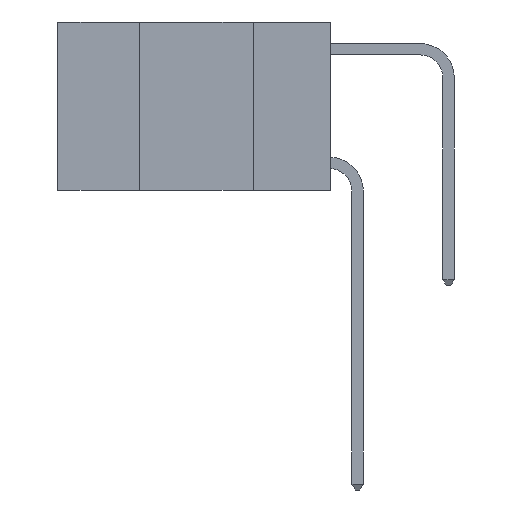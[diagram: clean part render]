
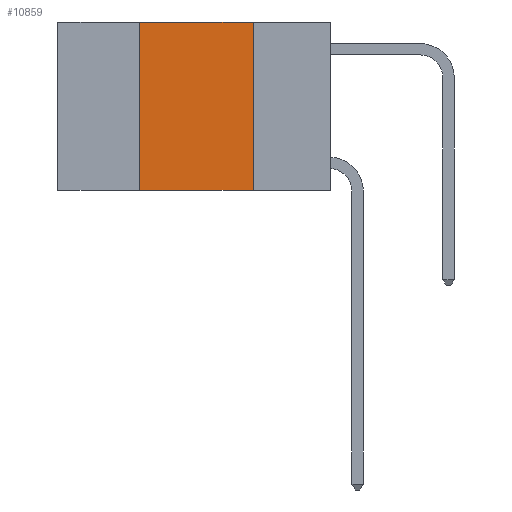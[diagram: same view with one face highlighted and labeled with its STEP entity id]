
A CAD part, left-side view. The second image highlights one B-rep face of the part: STEP entity #10859.
In plain terms, the highlighted planar face has unit normal (-1, 0, 0).
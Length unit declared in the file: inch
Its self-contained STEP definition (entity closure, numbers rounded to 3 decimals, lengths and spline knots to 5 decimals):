
#292 = DIRECTION ( 'NONE',  ( 0., -1., 0. ) ) ;
#1129 = CARTESIAN_POINT ( 'NONE',  ( 0., 0.6, 0. ) ) ;
#1498 = DIRECTION ( 'NONE',  ( 0., -1., 0. ) ) ;
#1882 = VERTEX_POINT ( 'NONE', #3026 ) ;
#1991 = CARTESIAN_POINT ( 'NONE',  ( 0., 0.17, 0. ) ) ;
#2131 = VECTOR ( 'NONE', #7748, 39.37008 ) ;
#3026 = CARTESIAN_POINT ( 'NONE',  ( 0., 0.17, -0.37 ) ) ;
#3060 = VERTEX_POINT ( 'NONE', #3488 ) ;
#3488 = CARTESIAN_POINT ( 'NONE',  ( 0., 0.42, 0. ) ) ;
#3491 = EDGE_CURVE ( 'NONE', #3060, #4662, #6987, .T. ) ;
#3756 = VECTOR ( 'NONE', #1498, 39.37008 ) ;
#3855 = FACE_OUTER_BOUND ( 'NONE', #8008, .T. ) ;
#4045 = LINE ( 'NONE', #7292, #3756 ) ;
#4110 = DIRECTION ( 'NONE',  ( 1., 0., 0. ) ) ;
#4662 = VERTEX_POINT ( 'NONE', #11612 ) ;
#4726 = VERTEX_POINT ( 'NONE', #6055 ) ;
#4732 = LINE ( 'NONE', #1991, #2131 ) ;
#5241 = ORIENTED_EDGE ( 'NONE', *, *, #9374, .T. ) ;
#5660 = ORIENTED_EDGE ( 'NONE', *, *, #5983, .F. ) ;
#5716 = EDGE_CURVE ( 'NONE', #4662, #1882, #4732, .T. ) ;
#5983 = EDGE_CURVE ( 'NONE', #4726, #3060, #10655, .T. ) ;
#6055 = CARTESIAN_POINT ( 'NONE',  ( 0., 0.42, -0.37 ) ) ;
#6681 = ORIENTED_EDGE ( 'NONE', *, *, #3491, .F. ) ;
#6701 = VECTOR ( 'NONE', #292, 39.37008 ) ;
#6905 = AXIS2_PLACEMENT_3D ( 'NONE', #1129, #4110, #10753 ) ;
#6987 = LINE ( 'NONE', #8049, #6701 ) ;
#7124 = ORIENTED_EDGE ( 'NONE', *, *, #5716, .F. ) ;
#7292 = CARTESIAN_POINT ( 'NONE',  ( 0., 0.6, -0.37 ) ) ;
#7547 = VECTOR ( 'NONE', #10938, 39.37008 ) ;
#7748 = DIRECTION ( 'NONE',  ( 0., 0., -1. ) ) ;
#8008 = EDGE_LOOP ( 'NONE', ( #7124, #6681, #5660, #5241 ) ) ;
#8049 = CARTESIAN_POINT ( 'NONE',  ( 0., 0.6, 0. ) ) ;
#8116 = CARTESIAN_POINT ( 'NONE',  ( 0., 0.42, 0. ) ) ;
#9374 = EDGE_CURVE ( 'NONE', #4726, #1882, #4045, .T. ) ;
#10655 = LINE ( 'NONE', #8116, #7547 ) ;
#10714 = PLANE ( 'NONE',  #6905 ) ;
#10753 = DIRECTION ( 'NONE',  ( 0., 0., -1. ) ) ;
#10859 = ADVANCED_FACE ( 'NONE', ( #3855 ), #10714, .F. ) ;
#10938 = DIRECTION ( 'NONE',  ( 0., 0., 1. ) ) ;
#11612 = CARTESIAN_POINT ( 'NONE',  ( 0., 0.17, 0. ) ) ;
